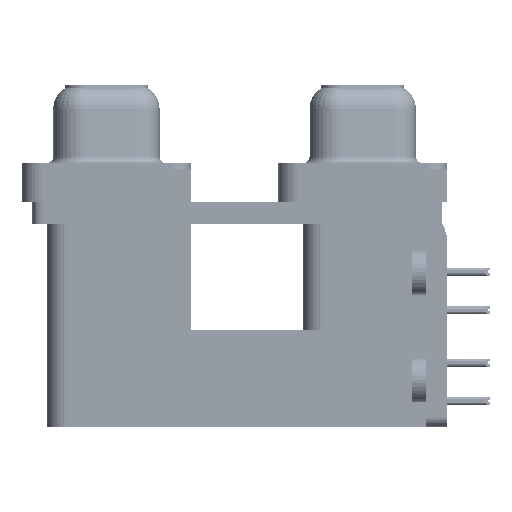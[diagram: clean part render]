
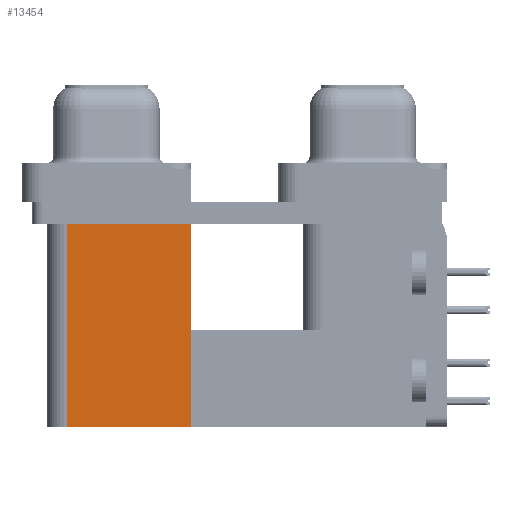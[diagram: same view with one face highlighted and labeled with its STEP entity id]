
A CAD part, left-side view. The second image highlights one B-rep face of the part: STEP entity #13454.
In plain terms, the highlighted planar face has unit normal (-1, 0, 0).
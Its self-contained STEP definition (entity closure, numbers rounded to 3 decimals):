
#2170 = CARTESIAN_POINT ( 'NONE',  ( 3.79, 12.775, -2.5 ) ) ;
#3663 = EDGE_CURVE ( 'NONE', #62788, #12583, #66508, .T. ) ;
#3888 = AXIS2_PLACEMENT_3D ( 'NONE', #32408, #13427, #14577 ) ;
#4060 = VERTEX_POINT ( 'NONE', #58955 ) ;
#4140 = EDGE_CURVE ( 'NONE', #12583, #26669, #27013, .T. ) ;
#5890 = ORIENTED_EDGE ( 'NONE', *, *, #46147, .F. ) ;
#5969 = VECTOR ( 'NONE', #73494, 1000. ) ;
#12583 = VERTEX_POINT ( 'NONE', #64583 ) ;
#13427 = DIRECTION ( 'NONE',  ( 1., 0., 0. ) ) ;
#13454 = ADVANCED_FACE ( 'NONE', ( #26211 ), #44471, .F. ) ;
#14163 = EDGE_CURVE ( 'NONE', #4060, #26669, #30825, .T. ) ;
#14225 = DIRECTION ( 'NONE',  ( 0., 1., 0. ) ) ;
#14577 = DIRECTION ( 'NONE',  ( 0., 0., -1. ) ) ;
#26042 = LINE ( 'NONE', #49762, #5969 ) ;
#26211 = FACE_OUTER_BOUND ( 'NONE', #54594, .T. ) ;
#26669 = VERTEX_POINT ( 'NONE', #69803 ) ;
#27013 = LINE ( 'NONE', #2170, #57142 ) ;
#30342 = DIRECTION ( 'NONE',  ( 0., 0., 1. ) ) ;
#30825 = LINE ( 'NONE', #44022, #46169 ) ;
#32408 = CARTESIAN_POINT ( 'NONE',  ( 3.79, 12.775, -19.2 ) ) ;
#33472 = VECTOR ( 'NONE', #30342, 1000. ) ;
#34854 = CARTESIAN_POINT ( 'NONE',  ( 3.79, 12.775, -19.2 ) ) ;
#36948 = CARTESIAN_POINT ( 'NONE',  ( 3.79, 12.775, -19.2 ) ) ;
#44022 = CARTESIAN_POINT ( 'NONE',  ( 3.79, 21.975, -19.2 ) ) ;
#44471 = PLANE ( 'NONE',  #3888 ) ;
#46147 = EDGE_CURVE ( 'NONE', #62788, #4060, #26042, .T. ) ;
#46169 = VECTOR ( 'NONE', #72454, 1000. ) ;
#49762 = CARTESIAN_POINT ( 'NONE',  ( 3.79, 12.775, -19.2 ) ) ;
#54594 = EDGE_LOOP ( 'NONE', ( #64277, #66225, #5890, #68974 ) ) ;
#57142 = VECTOR ( 'NONE', #14225, 1000. ) ;
#58955 = CARTESIAN_POINT ( 'NONE',  ( 3.79, 21.975, -19.2 ) ) ;
#62788 = VERTEX_POINT ( 'NONE', #34854 ) ;
#64277 = ORIENTED_EDGE ( 'NONE', *, *, #4140, .T. ) ;
#64583 = CARTESIAN_POINT ( 'NONE',  ( 3.79, 12.775, -2.5 ) ) ;
#66225 = ORIENTED_EDGE ( 'NONE', *, *, #14163, .F. ) ;
#66508 = LINE ( 'NONE', #36948, #33472 ) ;
#68974 = ORIENTED_EDGE ( 'NONE', *, *, #3663, .T. ) ;
#69803 = CARTESIAN_POINT ( 'NONE',  ( 3.79, 21.975, -2.5 ) ) ;
#72454 = DIRECTION ( 'NONE',  ( 0., 0., 1. ) ) ;
#73494 = DIRECTION ( 'NONE',  ( 0., 1., 0. ) ) ;
